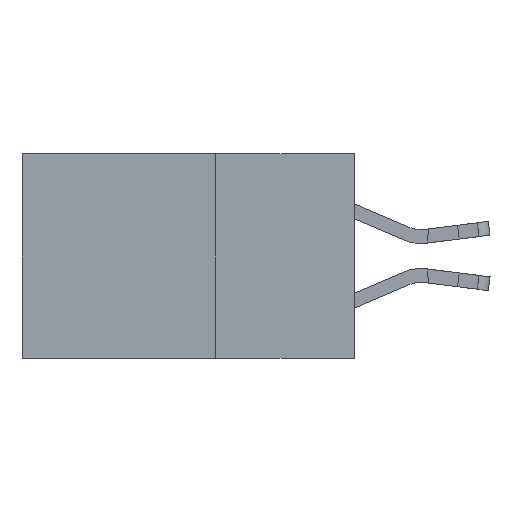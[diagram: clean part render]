
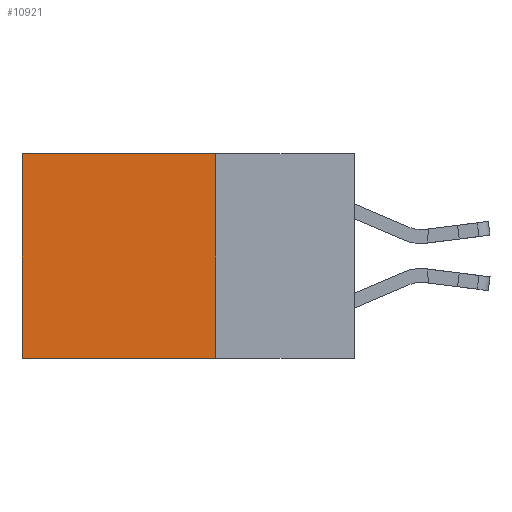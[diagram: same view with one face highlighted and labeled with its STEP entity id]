
A CAD part, left-side view. The second image highlights one B-rep face of the part: STEP entity #10921.
In plain terms, the highlighted planar face has unit normal (-1, 0, 0).
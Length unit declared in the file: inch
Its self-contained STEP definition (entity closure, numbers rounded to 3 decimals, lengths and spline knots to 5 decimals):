
#277 = ORIENTED_EDGE ( 'NONE', *, *, #12841, .F. ) ;
#378 = VERTEX_POINT ( 'NONE', #2383 ) ;
#918 = LINE ( 'NONE', #13185, #7392 ) ;
#1893 = VECTOR ( 'NONE', #18242, 39.37008 ) ;
#2383 = CARTESIAN_POINT ( 'NONE',  ( 0.2615, 0.6, 0. ) ) ;
#2738 = LINE ( 'NONE', #10890, #3670 ) ;
#3670 = VECTOR ( 'NONE', #12389, 39.37008 ) ;
#4506 = CARTESIAN_POINT ( 'NONE',  ( 0.2615, 0.25, -0.37 ) ) ;
#6070 = PLANE ( 'NONE',  #18568 ) ;
#6169 = CARTESIAN_POINT ( 'NONE',  ( 0.2615, 0.6, -0.37 ) ) ;
#6264 = ORIENTED_EDGE ( 'NONE', *, *, #18406, .T. ) ;
#6419 = VERTEX_POINT ( 'NONE', #17975 ) ;
#7149 = EDGE_CURVE ( 'NONE', #378, #9533, #15518, .T. ) ;
#7392 = VECTOR ( 'NONE', #14692, 39.37008 ) ;
#7541 = DIRECTION ( 'NONE',  ( 0., 0., -1. ) ) ;
#7910 = CARTESIAN_POINT ( 'NONE',  ( 0.2615, 0.25, -0.37 ) ) ;
#9533 = VERTEX_POINT ( 'NONE', #6169 ) ;
#10890 = CARTESIAN_POINT ( 'NONE',  ( 0.2615, 0.25, 0. ) ) ;
#10921 = ADVANCED_FACE ( 'NONE', ( #16263 ), #6070, .F. ) ;
#11443 = ORIENTED_EDGE ( 'NONE', *, *, #17404, .F. ) ;
#11486 = EDGE_LOOP ( 'NONE', ( #16533, #277, #11443, #6264 ) ) ;
#11631 = CARTESIAN_POINT ( 'NONE',  ( 0.2615, 0.25, 0. ) ) ;
#12389 = DIRECTION ( 'NONE',  ( 0., 1., 0. ) ) ;
#12841 = EDGE_CURVE ( 'NONE', #6419, #9533, #17132, .T. ) ;
#13185 = CARTESIAN_POINT ( 'NONE',  ( 0.2615, 0.25, -0.37 ) ) ;
#13616 = DIRECTION ( 'NONE',  ( 0., 0., -1. ) ) ;
#14692 = DIRECTION ( 'NONE',  ( 0., 0., -1. ) ) ;
#15518 = LINE ( 'NONE', #16473, #18982 ) ;
#16263 = FACE_OUTER_BOUND ( 'NONE', #11486, .T. ) ;
#16373 = DIRECTION ( 'NONE',  ( 1., 0., 0. ) ) ;
#16473 = CARTESIAN_POINT ( 'NONE',  ( 0.2615, 0.6, -0.37 ) ) ;
#16533 = ORIENTED_EDGE ( 'NONE', *, *, #7149, .T. ) ;
#17132 = LINE ( 'NONE', #7910, #1893 ) ;
#17375 = VERTEX_POINT ( 'NONE', #11631 ) ;
#17404 = EDGE_CURVE ( 'NONE', #17375, #6419, #918, .T. ) ;
#17975 = CARTESIAN_POINT ( 'NONE',  ( 0.2615, 0.25, -0.37 ) ) ;
#18242 = DIRECTION ( 'NONE',  ( 0., 1., 0. ) ) ;
#18406 = EDGE_CURVE ( 'NONE', #17375, #378, #2738, .T. ) ;
#18568 = AXIS2_PLACEMENT_3D ( 'NONE', #4506, #16373, #7541 ) ;
#18982 = VECTOR ( 'NONE', #13616, 39.37008 ) ;
